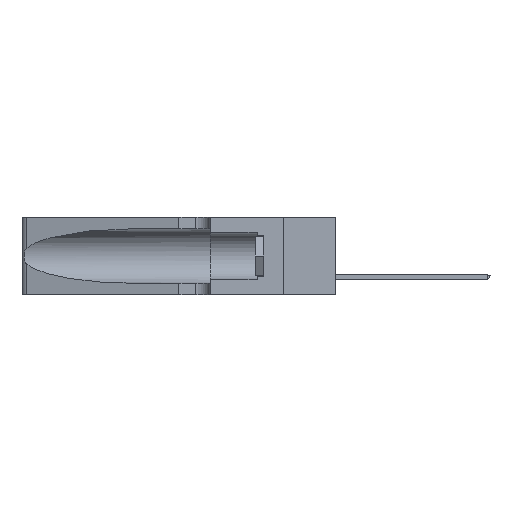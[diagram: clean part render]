
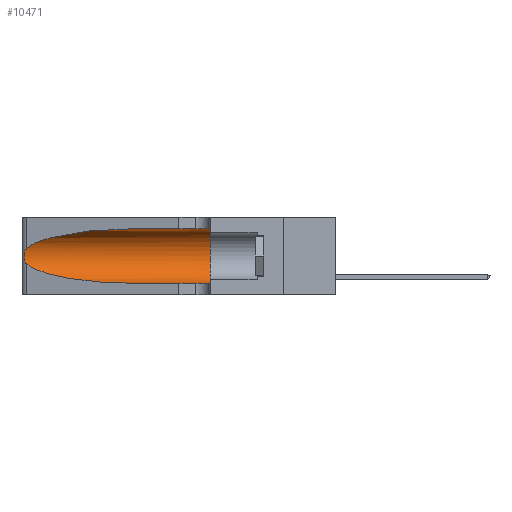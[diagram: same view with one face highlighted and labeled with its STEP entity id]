
A CAD part, left-side view. The second image highlights one B-rep face of the part: STEP entity #10471.
In plain terms, the highlighted cylindrical face has radius 3.308 mm (diameter 6.617 mm), a partial arc.
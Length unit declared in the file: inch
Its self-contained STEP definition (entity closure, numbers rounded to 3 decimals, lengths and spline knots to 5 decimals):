
#169 = DIRECTION ( 'NONE',  ( 0., 0., -1. ) ) ;
#213 = CARTESIAN_POINT ( 'NONE',  ( 0.25854, 1.2359, 0.20912 ) ) ;
#306 = CARTESIAN_POINT ( 'NONE',  ( 0.25639, 1.23186, 0.15144 ) ) ;
#594 = LINE ( 'NONE', #6024, #23465 ) ;
#1179 = VERTEX_POINT ( 'NONE', #16904 ) ;
#1466 = CARTESIAN_POINT ( 'NONE',  ( 0.18966, 0.96281, 0.05475 ) ) ;
#1559 = CARTESIAN_POINT ( 'NONE',  ( 0.25487, 1.22718, 0.14631 ) ) ;
#1981 = DIRECTION ( 'NONE',  ( 0., 1., 0. ) ) ;
#2427 = CARTESIAN_POINT ( 'NONE',  ( 0.25555, 1.22994, 0.2215 ) ) ;
#2616 = ORIENTED_EDGE ( 'NONE', *, *, #13591, .T. ) ;
#3544 = DIRECTION ( 'NONE',  ( 0., -1., 0. ) ) ;
#4112 = ORIENTED_EDGE ( 'NONE', *, *, #24113, .T. ) ;
#4465 = CARTESIAN_POINT ( 'NONE',  ( 0.26017, 1.23833, 0.17102 ) ) ;
#4528 = AXIS2_PLACEMENT_3D ( 'NONE', #10441, #19079, #169 ) ;
#4623 = VERTEX_POINT ( 'NONE', #6633 ) ;
#4626 =( BOUNDED_CURVE ( )  B_SPLINE_CURVE ( 3, ( #1559, #12121, #1466, #22501 ),
 .UNSPECIFIED., .F., .T. ) 
 B_SPLINE_CURVE_WITH_KNOTS ( ( 4, 4 ),
 ( 3.44316, 4.71239 ),
 .UNSPECIFIED. ) 
 CURVE ( )  GEOMETRIC_REPRESENTATION_ITEM ( )  RATIONAL_B_SPLINE_CURVE ( ( 1., 0.87, 0.87, 1. ) ) 
 REPRESENTATION_ITEM ( '' )  );
#4655 = CARTESIAN_POINT ( 'NONE',  ( 0.25487, 1.22718, 0.22369 ) ) ;
#4824 = CARTESIAN_POINT ( 'NONE',  ( 0.2373, 1.15595, 0.28018 ) ) ;
#5703 = ORIENTED_EDGE ( 'NONE', *, *, #23025, .F. ) ;
#6024 = CARTESIAN_POINT ( 'NONE',  ( 0.1305, 1.61858, 0.05475 ) ) ;
#6307 = CARTESIAN_POINT ( 'NONE',  ( 0.1305, 0.35, 0.05475 ) ) ;
#6616 = CARTESIAN_POINT ( 'NONE',  ( 0.25555, 1.22993, 0.14849 ) ) ;
#6633 = CARTESIAN_POINT ( 'NONE',  ( 0.25487, 1.22718, 0.22369 ) ) ;
#6804 = ORIENTED_EDGE ( 'NONE', *, *, #25422, .F. ) ;
#6897 = ORIENTED_EDGE ( 'NONE', *, *, #27369, .T. ) ;
#8190 = CARTESIAN_POINT ( 'NONE',  ( 0.1305, 0.35, 0.185 ) ) ;
#9092 = CARTESIAN_POINT ( 'NONE',  ( 0.25487, 1.22718, 0.22369 ) ) ;
#9993 = VERTEX_POINT ( 'NONE', #19557 ) ;
#10441 = CARTESIAN_POINT ( 'NONE',  ( 0.1305, 1.61858, 0.185 ) ) ;
#10471 = ADVANCED_FACE ( 'NONE', ( #10688 ), #13041, .F. ) ;
#10569 = VERTEX_POINT ( 'NONE', #24337 ) ;
#10682 = DIRECTION ( 'NONE',  ( 0., 0., 1. ) ) ;
#10688 = FACE_OUTER_BOUND ( 'NONE', #21138, .T. ) ;
#10864 = CARTESIAN_POINT ( 'NONE',  ( 0.26018, 1.23835, 0.19895 ) ) ;
#11685 = ORIENTED_EDGE ( 'NONE', *, *, #21816, .T. ) ;
#12121 = CARTESIAN_POINT ( 'NONE',  ( 0.2373, 1.15595, 0.08982 ) ) ;
#13041 = CYLINDRICAL_SURFACE ( 'NONE', #4528, 0.13025 ) ;
#13275 = CARTESIAN_POINT ( 'NONE',  ( 0.18966, 0.96281, 0.31525 ) ) ;
#13591 = EDGE_CURVE ( 'NONE', #1179, #4623, #26673, .T. ) ;
#14135 = B_SPLINE_CURVE_WITH_KNOTS ( 'NONE', 3,
 ( #4655, #2427, #23639, #21341, #213, #10864, #19503, #17186, #4465, #19311, #15330, #306, #6616, #15142 ),
 .UNSPECIFIED., .F., .F.,
 ( 4, 2, 2, 2, 2, 2, 4 ),
 ( 0., 0.00027, 0.00053, 0.00107, 0.0016, 0.00187, 0.00214 ),
 .UNSPECIFIED. ) ;
#15142 = CARTESIAN_POINT ( 'NONE',  ( 0.25487, 1.22718, 0.14631 ) ) ;
#15330 = CARTESIAN_POINT ( 'NONE',  ( 0.25789, 1.23486, 0.15765 ) ) ;
#15401 = CARTESIAN_POINT ( 'NONE',  ( 0.1305, 0.72297, 0.31525 ) ) ;
#16497 = DIRECTION ( 'NONE',  ( 0., -1., 0. ) ) ;
#16904 = CARTESIAN_POINT ( 'NONE',  ( 0.1305, 0.72297, 0.31525 ) ) ;
#17006 = AXIS2_PLACEMENT_3D ( 'NONE', #8190, #1981, #10682 ) ;
#17186 = CARTESIAN_POINT ( 'NONE',  ( 0.26075, 1.23896, 0.178 ) ) ;
#17639 = LINE ( 'NONE', #20780, #21919 ) ;
#18734 = CIRCLE ( 'NONE', #17006, 0.13025 ) ;
#19079 = DIRECTION ( 'NONE',  ( 0., -1., 0. ) ) ;
#19311 = CARTESIAN_POINT ( 'NONE',  ( 0.25856, 1.23593, 0.16098 ) ) ;
#19503 = CARTESIAN_POINT ( 'NONE',  ( 0.26075, 1.23896, 0.19203 ) ) ;
#19557 = CARTESIAN_POINT ( 'NONE',  ( 0.25487, 1.22718, 0.14631 ) ) ;
#20318 = VERTEX_POINT ( 'NONE', #22756 ) ;
#20780 = CARTESIAN_POINT ( 'NONE',  ( 0.1305, 1.61858, 0.31525 ) ) ;
#21138 = EDGE_LOOP ( 'NONE', ( #2616, #6897, #4112, #11685, #5703, #6804 ) ) ;
#21341 = CARTESIAN_POINT ( 'NONE',  ( 0.25787, 1.23484, 0.2124 ) ) ;
#21769 = VERTEX_POINT ( 'NONE', #6307 ) ;
#21816 = EDGE_CURVE ( 'NONE', #20318, #21769, #594, .T. ) ;
#21919 = VECTOR ( 'NONE', #3544, 39.37008 ) ;
#22501 = CARTESIAN_POINT ( 'NONE',  ( 0.1305, 0.72297, 0.05475 ) ) ;
#22756 = CARTESIAN_POINT ( 'NONE',  ( 0.1305, 0.72297, 0.05475 ) ) ;
#23025 = EDGE_CURVE ( 'NONE', #10569, #21769, #18734, .T. ) ;
#23465 = VECTOR ( 'NONE', #16497, 39.37008 ) ;
#23639 = CARTESIAN_POINT ( 'NONE',  ( 0.25639, 1.23184, 0.21858 ) ) ;
#24113 = EDGE_CURVE ( 'NONE', #9993, #20318, #4626, .T. ) ;
#24337 = CARTESIAN_POINT ( 'NONE',  ( 0.1305, 0.35, 0.31525 ) ) ;
#25422 = EDGE_CURVE ( 'NONE', #1179, #10569, #17639, .T. ) ;
#26673 =( BOUNDED_CURVE ( )  B_SPLINE_CURVE ( 3, ( #15401, #13275, #4824, #9092 ),
 .UNSPECIFIED., .F., .F. ) 
 B_SPLINE_CURVE_WITH_KNOTS ( ( 4, 4 ),
 ( 1.5708, 2.84003 ),
 .UNSPECIFIED. ) 
 CURVE ( )  GEOMETRIC_REPRESENTATION_ITEM ( )  RATIONAL_B_SPLINE_CURVE ( ( 1., 0.87, 0.87, 1. ) ) 
 REPRESENTATION_ITEM ( '' )  );
#27369 = EDGE_CURVE ( 'NONE', #4623, #9993, #14135, .T. ) ;
